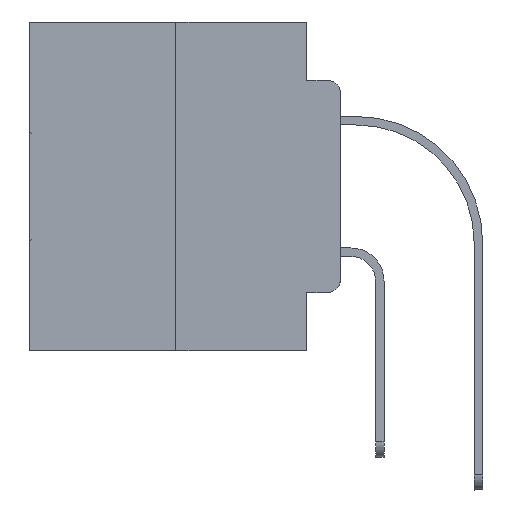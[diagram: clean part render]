
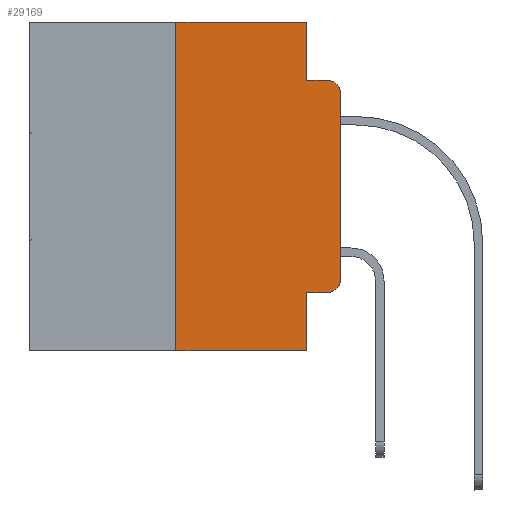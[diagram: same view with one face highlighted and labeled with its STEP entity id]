
A CAD part, left-side view. The second image highlights one B-rep face of the part: STEP entity #29169.
In plain terms, the highlighted planar face has unit normal (-1, 0, 0).
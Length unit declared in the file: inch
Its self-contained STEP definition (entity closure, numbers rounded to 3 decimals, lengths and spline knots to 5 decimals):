
#45 = DIRECTION ( 'NONE',  ( 0., -1., 0. ) ) ;
#107 = VERTEX_POINT ( 'NONE', #22052 ) ;
#384 = DIRECTION ( 'NONE',  ( -1., 0., 0. ) ) ;
#394 = AXIS2_PLACEMENT_3D ( 'NONE', #15883, #2818, #25694 ) ;
#770 = CARTESIAN_POINT ( 'NONE',  ( 0., 0.473, 0. ) ) ;
#871 = CARTESIAN_POINT ( 'NONE',  ( 0., 0.051, 0. ) ) ;
#959 = LINE ( 'NONE', #6482, #31156 ) ;
#2088 = DIRECTION ( 'NONE',  ( -1., 0., 0. ) ) ;
#2283 = LINE ( 'NONE', #14703, #22775 ) ;
#2818 = DIRECTION ( 'NONE',  ( 1., 0., 0. ) ) ;
#2972 = CARTESIAN_POINT ( 'NONE',  ( 0., 0.051, 0. ) ) ;
#3132 = DIRECTION ( 'NONE',  ( 0., 0., -1. ) ) ;
#3576 = EDGE_LOOP ( 'NONE', ( #22102, #27338, #6209, #5410, #27824, #5158, #26195, #28278, #21953, #31491 ) ) ;
#3634 = EDGE_CURVE ( 'NONE', #27156, #30779, #22631, .T. ) ;
#3889 = EDGE_CURVE ( 'NONE', #19049, #21469, #6250, .T. ) ;
#4978 = CIRCLE ( 'NONE', #25835, 0.02 ) ;
#5158 = ORIENTED_EDGE ( 'NONE', *, *, #3634, .F. ) ;
#5410 = ORIENTED_EDGE ( 'NONE', *, *, #3889, .F. ) ;
#5887 = LINE ( 'NONE', #2972, #7474 ) ;
#6042 = VECTOR ( 'NONE', #30827, 39.37008 ) ;
#6067 = VECTOR ( 'NONE', #30683, 39.37008 ) ;
#6209 = ORIENTED_EDGE ( 'NONE', *, *, #15196, .F. ) ;
#6250 = LINE ( 'NONE', #871, #6042 ) ;
#6482 = CARTESIAN_POINT ( 'NONE',  ( 0., 0.051, -0.4115 ) ) ;
#7471 = CARTESIAN_POINT ( 'NONE',  ( 0., 0.051, -0.4115 ) ) ;
#7474 = VECTOR ( 'NONE', #3132, 39.37008 ) ;
#8212 = VECTOR ( 'NONE', #20746, 39.37008 ) ;
#8416 = VERTEX_POINT ( 'NONE', #10010 ) ;
#9772 = DIRECTION ( 'NONE',  ( 0., 0., -1. ) ) ;
#10010 = CARTESIAN_POINT ( 'NONE',  ( 0., 0.051, -0.5 ) ) ;
#10170 = FACE_OUTER_BOUND ( 'NONE', #3576, .T. ) ;
#10339 = CARTESIAN_POINT ( 'NONE',  ( 0., 0.02, -0.1085 ) ) ;
#10669 = CARTESIAN_POINT ( 'NONE',  ( 0., 0.051, -0.0885 ) ) ;
#11788 = VERTEX_POINT ( 'NONE', #13671 ) ;
#11937 = EDGE_CURVE ( 'NONE', #30779, #19049, #13202, .T. ) ;
#12248 = DIRECTION ( 'NONE',  ( 0., 0., 1. ) ) ;
#12466 = CARTESIAN_POINT ( 'NONE',  ( 0., 0.473, -0.5 ) ) ;
#13024 = EDGE_CURVE ( 'NONE', #17891, #26065, #959, .T. ) ;
#13202 = LINE ( 'NONE', #770, #8212 ) ;
#13671 = CARTESIAN_POINT ( 'NONE',  ( 0., 0.02, -0.0885 ) ) ;
#14703 = CARTESIAN_POINT ( 'NONE',  ( 0., 0., 0. ) ) ;
#15196 = EDGE_CURVE ( 'NONE', #21469, #11788, #28220, .T. ) ;
#15197 = CARTESIAN_POINT ( 'NONE',  ( 0., 0., -0.1085 ) ) ;
#15264 = CARTESIAN_POINT ( 'NONE',  ( 0., 0.25, 0. ) ) ;
#15883 = CARTESIAN_POINT ( 'NONE',  ( 0., 0.473, 0. ) ) ;
#16159 = DIRECTION ( 'NONE',  ( 0., -1., 0. ) ) ;
#16994 = EDGE_CURVE ( 'NONE', #17891, #8416, #5887, .T. ) ;
#17149 = CARTESIAN_POINT ( 'NONE',  ( 0., 0.051, 0. ) ) ;
#17472 = CIRCLE ( 'NONE', #32113, 0.02 ) ;
#17479 = VERTEX_POINT ( 'NONE', #15197 ) ;
#17891 = VERTEX_POINT ( 'NONE', #7471 ) ;
#17921 = CARTESIAN_POINT ( 'NONE',  ( 0., 0.051, -0.0885 ) ) ;
#18592 = VECTOR ( 'NONE', #30010, 39.37008 ) ;
#18826 = EDGE_CURVE ( 'NONE', #27156, #8416, #30325, .T. ) ;
#19049 = VERTEX_POINT ( 'NONE', #17149 ) ;
#20746 = DIRECTION ( 'NONE',  ( 0., -1., 0. ) ) ;
#21469 = VERTEX_POINT ( 'NONE', #17921 ) ;
#21953 = ORIENTED_EDGE ( 'NONE', *, *, #13024, .T. ) ;
#22052 = CARTESIAN_POINT ( 'NONE',  ( 0., 0., -0.3915 ) ) ;
#22102 = ORIENTED_EDGE ( 'NONE', *, *, #26255, .T. ) ;
#22167 = CARTESIAN_POINT ( 'NONE',  ( 0., 0.25, -0.5 ) ) ;
#22631 = LINE ( 'NONE', #15264, #18592 ) ;
#22775 = VECTOR ( 'NONE', #12248, 39.37008 ) ;
#23102 = PLANE ( 'NONE',  #394 ) ;
#24493 = CARTESIAN_POINT ( 'NONE',  ( 0., 0.02, -0.3915 ) ) ;
#25556 = EDGE_CURVE ( 'NONE', #26065, #107, #4978, .T. ) ;
#25694 = DIRECTION ( 'NONE',  ( 0., 0., -1. ) ) ;
#25835 = AXIS2_PLACEMENT_3D ( 'NONE', #24493, #2088, #9772 ) ;
#26065 = VERTEX_POINT ( 'NONE', #28005 ) ;
#26195 = ORIENTED_EDGE ( 'NONE', *, *, #18826, .T. ) ;
#26255 = EDGE_CURVE ( 'NONE', #107, #17479, #2283, .T. ) ;
#27156 = VERTEX_POINT ( 'NONE', #22167 ) ;
#27338 = ORIENTED_EDGE ( 'NONE', *, *, #31249, .T. ) ;
#27824 = ORIENTED_EDGE ( 'NONE', *, *, #11937, .F. ) ;
#28005 = CARTESIAN_POINT ( 'NONE',  ( 0., 0.02, -0.4115 ) ) ;
#28220 = LINE ( 'NONE', #10669, #6067 ) ;
#28278 = ORIENTED_EDGE ( 'NONE', *, *, #16994, .F. ) ;
#29169 = ADVANCED_FACE ( 'NONE', ( #10170 ), #23102, .F. ) ;
#29621 = VECTOR ( 'NONE', #45, 39.37008 ) ;
#29726 = CARTESIAN_POINT ( 'NONE',  ( 0., 0.25, 0. ) ) ;
#30000 = DIRECTION ( 'NONE',  ( 0., 0., -1. ) ) ;
#30010 = DIRECTION ( 'NONE',  ( 0., 0., 1. ) ) ;
#30325 = LINE ( 'NONE', #12466, #29621 ) ;
#30683 = DIRECTION ( 'NONE',  ( 0., -1., 0. ) ) ;
#30779 = VERTEX_POINT ( 'NONE', #29726 ) ;
#30827 = DIRECTION ( 'NONE',  ( 0., 0., -1. ) ) ;
#31156 = VECTOR ( 'NONE', #16159, 39.37008 ) ;
#31249 = EDGE_CURVE ( 'NONE', #17479, #11788, #17472, .T. ) ;
#31491 = ORIENTED_EDGE ( 'NONE', *, *, #25556, .T. ) ;
#32113 = AXIS2_PLACEMENT_3D ( 'NONE', #10339, #384, #30000 ) ;
